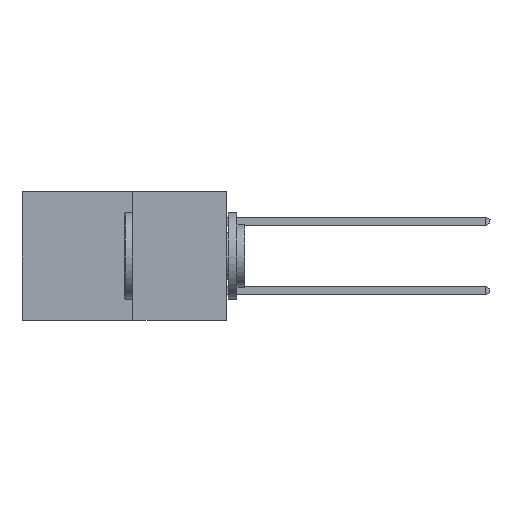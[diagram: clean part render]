
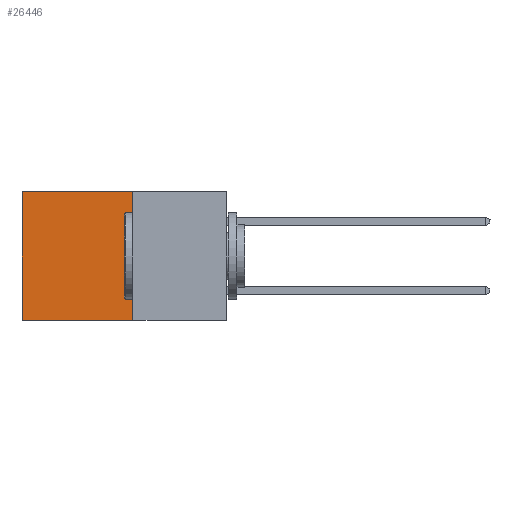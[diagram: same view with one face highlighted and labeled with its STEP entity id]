
A CAD part, left-side view. The second image highlights one B-rep face of the part: STEP entity #26446.
In plain terms, the highlighted planar face has unit normal (-1, 0, 0).
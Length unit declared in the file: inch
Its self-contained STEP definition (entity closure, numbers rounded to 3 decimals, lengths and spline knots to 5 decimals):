
#1383 = CARTESIAN_POINT ( 'NONE',  ( 0.277, 0.59, 0. ) ) ;
#1967 = CARTESIAN_POINT ( 'NONE',  ( 0.277, 0.27, -0.37 ) ) ;
#2446 = VERTEX_POINT ( 'NONE', #1967 ) ;
#2606 = CARTESIAN_POINT ( 'NONE',  ( 0.277, 0.27, 0. ) ) ;
#2660 = LINE ( 'NONE', #23725, #20862 ) ;
#4792 = AXIS2_PLACEMENT_3D ( 'NONE', #31000, #14883, #33694 ) ;
#4824 = DIRECTION ( 'NONE',  ( 0., 1., 0. ) ) ;
#6152 = EDGE_CURVE ( 'NONE', #32968, #2446, #18209, .T. ) ;
#6743 = PLANE ( 'NONE',  #4792 ) ;
#7686 = DIRECTION ( 'NONE',  ( 0., 0., -1. ) ) ;
#7740 = CARTESIAN_POINT ( 'NONE',  ( 0.277, 0.27, 0. ) ) ;
#9335 = VECTOR ( 'NONE', #27337, 39.37008 ) ;
#11178 = VERTEX_POINT ( 'NONE', #1383 ) ;
#11729 = LINE ( 'NONE', #7740, #12585 ) ;
#11893 = ORIENTED_EDGE ( 'NONE', *, *, #20078, .F. ) ;
#12585 = VECTOR ( 'NONE', #29317, 39.37008 ) ;
#12633 = ORIENTED_EDGE ( 'NONE', *, *, #31426, .T. ) ;
#13490 = ORIENTED_EDGE ( 'NONE', *, *, #14981, .T. ) ;
#13853 = CARTESIAN_POINT ( 'NONE',  ( 0.277, 0.59, -0.37 ) ) ;
#13856 = VERTEX_POINT ( 'NONE', #20112 ) ;
#14883 = DIRECTION ( 'NONE',  ( 1., 0., 0. ) ) ;
#14981 = EDGE_CURVE ( 'NONE', #11178, #13856, #26286, .T. ) ;
#16605 = ORIENTED_EDGE ( 'NONE', *, *, #6152, .F. ) ;
#17347 = VECTOR ( 'NONE', #7686, 39.37008 ) ;
#18209 = LINE ( 'NONE', #23932, #17347 ) ;
#20078 = EDGE_CURVE ( 'NONE', #2446, #13856, #2660, .T. ) ;
#20112 = CARTESIAN_POINT ( 'NONE',  ( 0.277, 0.59, -0.37 ) ) ;
#20862 = VECTOR ( 'NONE', #4824, 39.37008 ) ;
#23725 = CARTESIAN_POINT ( 'NONE',  ( 0.277, 0.27, -0.37 ) ) ;
#23932 = CARTESIAN_POINT ( 'NONE',  ( 0.277, 0.27, -0.37 ) ) ;
#26286 = LINE ( 'NONE', #13853, #9335 ) ;
#26446 = ADVANCED_FACE ( 'NONE', ( #34405 ), #6743, .F. ) ;
#27337 = DIRECTION ( 'NONE',  ( 0., 0., -1. ) ) ;
#27822 = EDGE_LOOP ( 'NONE', ( #13490, #11893, #16605, #12633 ) ) ;
#29317 = DIRECTION ( 'NONE',  ( 0., 1., 0. ) ) ;
#31000 = CARTESIAN_POINT ( 'NONE',  ( 0.277, 0.27, -0.37 ) ) ;
#31426 = EDGE_CURVE ( 'NONE', #32968, #11178, #11729, .T. ) ;
#32968 = VERTEX_POINT ( 'NONE', #2606 ) ;
#33694 = DIRECTION ( 'NONE',  ( 0., 0., -1. ) ) ;
#34405 = FACE_OUTER_BOUND ( 'NONE', #27822, .T. ) ;
